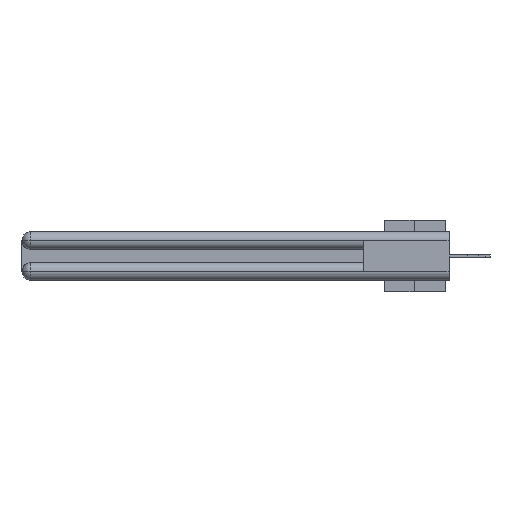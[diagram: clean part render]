
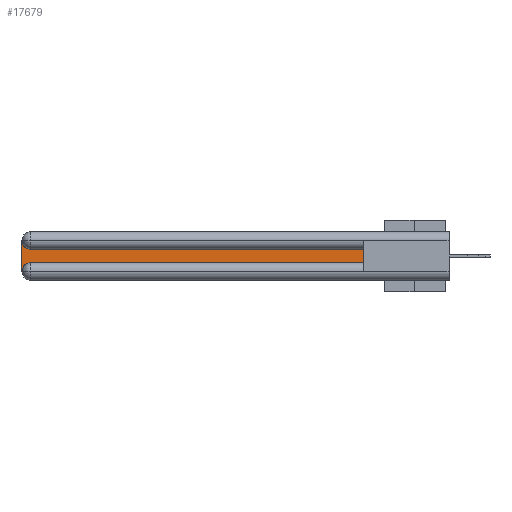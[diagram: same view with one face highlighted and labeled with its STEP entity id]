
A CAD part, left-side view. The second image highlights one B-rep face of the part: STEP entity #17679.
In plain terms, the highlighted planar face has unit normal (-1, 0, 0).
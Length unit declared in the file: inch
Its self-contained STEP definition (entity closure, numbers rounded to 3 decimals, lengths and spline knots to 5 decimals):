
#860 = ORIENTED_EDGE ( 'NONE', *, *, #37799, .T. ) ;
#1501 = DIRECTION ( 'NONE',  ( 0., 0., -1. ) ) ;
#1697 = CARTESIAN_POINT ( 'NONE',  ( 0.075, 0.6, -0.2175 ) ) ;
#1991 = ORIENTED_EDGE ( 'NONE', *, *, #35585, .T. ) ;
#2400 = ORIENTED_EDGE ( 'NONE', *, *, #33924, .T. ) ;
#2507 = ORIENTED_EDGE ( 'NONE', *, *, #35369, .T. ) ;
#3147 = CARTESIAN_POINT ( 'NONE',  ( 0.075, 2.94, -0.1225 ) ) ;
#3562 = DIRECTION ( 'NONE',  ( 0., 0., -1. ) ) ;
#3871 = CARTESIAN_POINT ( 'NONE',  ( 0.075, 3., -0.0625 ) ) ;
#6431 = CARTESIAN_POINT ( 'NONE',  ( 0.075, 3., -0.1225 ) ) ;
#6483 = CARTESIAN_POINT ( 'NONE',  ( 0.075, 3., -0.2175 ) ) ;
#8273 = CARTESIAN_POINT ( 'NONE',  ( 0.075, 0.6, -0.1225 ) ) ;
#9085 = FACE_OUTER_BOUND ( 'NONE', #19887, .T. ) ;
#9772 = CARTESIAN_POINT ( 'NONE',  ( 0.075, 0.6, -0.1225 ) ) ;
#10786 = CARTESIAN_POINT ( 'NONE',  ( 0.075, 2.94, -0.2775 ) ) ;
#11222 = DIRECTION ( 'NONE',  ( 0., 1., 0. ) ) ;
#11452 = VERTEX_POINT ( 'NONE', #3147 ) ;
#13146 = EDGE_CURVE ( 'NONE', #20883, #15903, #19938, .T. ) ;
#13695 = CARTESIAN_POINT ( 'NONE',  ( 0.075, 0.6, -0.2175 ) ) ;
#13701 = DIRECTION ( 'NONE',  ( 0., 0., -1. ) ) ;
#15224 = PLANE ( 'NONE',  #19501 ) ;
#15706 = VERTEX_POINT ( 'NONE', #32120 ) ;
#15903 = VERTEX_POINT ( 'NONE', #9772 ) ;
#16487 = CIRCLE ( 'NONE', #29709, 0.06 ) ;
#17163 = VERTEX_POINT ( 'NONE', #3871 ) ;
#17679 = ADVANCED_FACE ( 'NONE', ( #9085 ), #15224, .F. ) ;
#19080 = DIRECTION ( 'NONE',  ( 1., 0., 0. ) ) ;
#19501 = AXIS2_PLACEMENT_3D ( 'NONE', #6431, #21121, #3562 ) ;
#19887 = EDGE_LOOP ( 'NONE', ( #2507, #2400, #1991, #860, #25702, #28464 ) ) ;
#19938 = LINE ( 'NONE', #13695, #35438 ) ;
#20883 = VERTEX_POINT ( 'NONE', #26022 ) ;
#21121 = DIRECTION ( 'NONE',  ( 1., 0., 0. ) ) ;
#22274 = DIRECTION ( 'NONE',  ( 0., -1., 0. ) ) ;
#22676 = CARTESIAN_POINT ( 'NONE',  ( 0.075, 2.94, -0.2175 ) ) ;
#24043 = DIRECTION ( 'NONE',  ( 0., 0., -1. ) ) ;
#25702 = ORIENTED_EDGE ( 'NONE', *, *, #36597, .T. ) ;
#26022 = CARTESIAN_POINT ( 'NONE',  ( 0.075, 0.6, -0.2175 ) ) ;
#26858 = CIRCLE ( 'NONE', #31315, 0.06 ) ;
#27286 = LINE ( 'NONE', #6483, #34919 ) ;
#27778 = LINE ( 'NONE', #8273, #34491 ) ;
#28464 = ORIENTED_EDGE ( 'NONE', *, *, #13146, .T. ) ;
#29709 = AXIS2_PLACEMENT_3D ( 'NONE', #10786, #31220, #13701 ) ;
#31220 = DIRECTION ( 'NONE',  ( 1., 0., 0. ) ) ;
#31253 = VECTOR ( 'NONE', #22274, 39.37008 ) ;
#31315 = AXIS2_PLACEMENT_3D ( 'NONE', #36545, #19080, #1501 ) ;
#32120 = CARTESIAN_POINT ( 'NONE',  ( 0.075, 3., -0.2775 ) ) ;
#33924 = EDGE_CURVE ( 'NONE', #11452, #17163, #26858, .T. ) ;
#34491 = VECTOR ( 'NONE', #11222, 39.37008 ) ;
#34717 = VERTEX_POINT ( 'NONE', #22676 ) ;
#34919 = VECTOR ( 'NONE', #24043, 39.37008 ) ;
#35369 = EDGE_CURVE ( 'NONE', #15903, #11452, #27778, .T. ) ;
#35438 = VECTOR ( 'NONE', #37032, 39.37008 ) ;
#35585 = EDGE_CURVE ( 'NONE', #17163, #15706, #27286, .T. ) ;
#36545 = CARTESIAN_POINT ( 'NONE',  ( 0.075, 2.94, -0.0625 ) ) ;
#36597 = EDGE_CURVE ( 'NONE', #34717, #20883, #37128, .T. ) ;
#37032 = DIRECTION ( 'NONE',  ( 0., 0., 1. ) ) ;
#37128 = LINE ( 'NONE', #1697, #31253 ) ;
#37799 = EDGE_CURVE ( 'NONE', #15706, #34717, #16487, .T. ) ;
